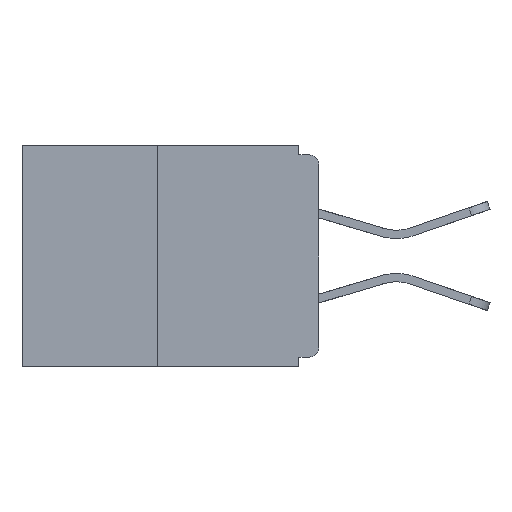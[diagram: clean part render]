
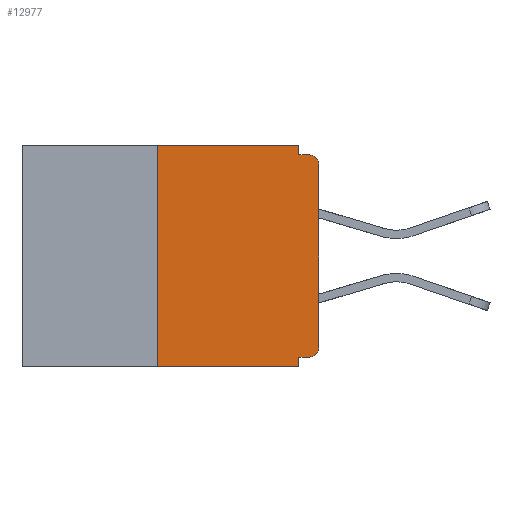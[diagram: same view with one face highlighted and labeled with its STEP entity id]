
A CAD part, left-side view. The second image highlights one B-rep face of the part: STEP entity #12977.
In plain terms, the highlighted planar face has unit normal (-1, 0, 0).
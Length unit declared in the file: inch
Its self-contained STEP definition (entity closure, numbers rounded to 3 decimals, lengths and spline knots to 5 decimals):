
#182 = DIRECTION ( 'NONE',  ( -1., 0., 0. ) ) ;
#202 = CIRCLE ( 'NONE', #8596, 0.015 ) ;
#263 = ORIENTED_EDGE ( 'NONE', *, *, #22919, .T. ) ;
#652 = VERTEX_POINT ( 'NONE', #20610 ) ;
#676 = VERTEX_POINT ( 'NONE', #3017 ) ;
#887 = CARTESIAN_POINT ( 'NONE',  ( 0., 0.031, -0.343 ) ) ;
#1121 = CARTESIAN_POINT ( 'NONE',  ( 0., 0.25, 0. ) ) ;
#1158 = CARTESIAN_POINT ( 'NONE',  ( 0., 0.031, -0.343 ) ) ;
#1607 = VERTEX_POINT ( 'NONE', #1121 ) ;
#2132 = DIRECTION ( 'NONE',  ( -1., 0., 0. ) ) ;
#2192 = VECTOR ( 'NONE', #4013, 39.37008 ) ;
#2248 = ORIENTED_EDGE ( 'NONE', *, *, #24231, .F. ) ;
#2489 = LINE ( 'NONE', #22765, #22977 ) ;
#2720 = VERTEX_POINT ( 'NONE', #15663 ) ;
#2823 = VERTEX_POINT ( 'NONE', #17191 ) ;
#3009 = DIRECTION ( 'NONE',  ( 0., 0., -1. ) ) ;
#3017 = CARTESIAN_POINT ( 'NONE',  ( 0., 0.031, -0.328 ) ) ;
#3618 = LINE ( 'NONE', #21144, #23528 ) ;
#4013 = DIRECTION ( 'NONE',  ( 0., 1., 0. ) ) ;
#4176 = DIRECTION ( 'NONE',  ( 0., -1., 0. ) ) ;
#4643 = VERTEX_POINT ( 'NONE', #14432 ) ;
#5268 = LINE ( 'NONE', #6237, #23670 ) ;
#5896 = ORIENTED_EDGE ( 'NONE', *, *, #14411, .F. ) ;
#6237 = CARTESIAN_POINT ( 'NONE',  ( 0., 0.031, 0. ) ) ;
#6320 = ORIENTED_EDGE ( 'NONE', *, *, #21836, .T. ) ;
#6542 = DIRECTION ( 'NONE',  ( 0., 0., -1. ) ) ;
#6616 = PLANE ( 'NONE',  #24752 ) ;
#7082 = LINE ( 'NONE', #15907, #23379 ) ;
#7353 = CARTESIAN_POINT ( 'NONE',  ( 0., 0.46, 0. ) ) ;
#7375 = VERTEX_POINT ( 'NONE', #23966 ) ;
#7377 = LINE ( 'NONE', #19166, #24196 ) ;
#7943 = DIRECTION ( 'NONE',  ( 0., 0., -1. ) ) ;
#7970 = EDGE_CURVE ( 'NONE', #4643, #1607, #2489, .T. ) ;
#8152 = LINE ( 'NONE', #1158, #17791 ) ;
#8422 = ORIENTED_EDGE ( 'NONE', *, *, #22274, .F. ) ;
#8554 = DIRECTION ( 'NONE',  ( 1., 0., 0. ) ) ;
#8596 = AXIS2_PLACEMENT_3D ( 'NONE', #21632, #2132, #7943 ) ;
#9411 = EDGE_CURVE ( 'NONE', #676, #18682, #8152, .T. ) ;
#10664 = VERTEX_POINT ( 'NONE', #11056 ) ;
#11056 = CARTESIAN_POINT ( 'NONE',  ( 0., 0., -0.03 ) ) ;
#11621 = ORIENTED_EDGE ( 'NONE', *, *, #9411, .F. ) ;
#11983 = FACE_OUTER_BOUND ( 'NONE', #19455, .T. ) ;
#12192 = CARTESIAN_POINT ( 'NONE',  ( 0., 0.015, -0.328 ) ) ;
#12699 = DIRECTION ( 'NONE',  ( 0., -1., 0. ) ) ;
#12977 = ADVANCED_FACE ( 'NONE', ( #11983 ), #6616, .F. ) ;
#13594 = DIRECTION ( 'NONE',  ( 0., -1., 0. ) ) ;
#13879 = DIRECTION ( 'NONE',  ( 0., 0., -1. ) ) ;
#14411 = EDGE_CURVE ( 'NONE', #1607, #2720, #22792, .T. ) ;
#14432 = CARTESIAN_POINT ( 'NONE',  ( 0., 0.25, -0.343 ) ) ;
#15440 = DIRECTION ( 'NONE',  ( 0., 0., 1. ) ) ;
#15663 = CARTESIAN_POINT ( 'NONE',  ( 0., 0.031, 0. ) ) ;
#15907 = CARTESIAN_POINT ( 'NONE',  ( 0., 0., -0.015 ) ) ;
#16020 = AXIS2_PLACEMENT_3D ( 'NONE', #17445, #182, #23494 ) ;
#17191 = CARTESIAN_POINT ( 'NONE',  ( 0., 0.015, -0.015 ) ) ;
#17396 = VECTOR ( 'NONE', #12699, 39.37008 ) ;
#17445 = CARTESIAN_POINT ( 'NONE',  ( 0., 0.015, -0.313 ) ) ;
#17791 = VECTOR ( 'NONE', #3009, 39.37008 ) ;
#18682 = VERTEX_POINT ( 'NONE', #887 ) ;
#19166 = CARTESIAN_POINT ( 'NONE',  ( 0., 0.46, -0.343 ) ) ;
#19455 = EDGE_LOOP ( 'NONE', ( #5896, #22480, #263, #11621, #2248, #20048, #23774, #6320, #20461, #8422 ) ) ;
#20048 = ORIENTED_EDGE ( 'NONE', *, *, #20972, .T. ) ;
#20402 = CIRCLE ( 'NONE', #16020, 0.015 ) ;
#20461 = ORIENTED_EDGE ( 'NONE', *, *, #22398, .F. ) ;
#20610 = CARTESIAN_POINT ( 'NONE',  ( 0., 0.031, -0.015 ) ) ;
#20972 = EDGE_CURVE ( 'NONE', #22016, #7375, #20402, .T. ) ;
#21144 = CARTESIAN_POINT ( 'NONE',  ( 0., 0., 0. ) ) ;
#21451 = CARTESIAN_POINT ( 'NONE',  ( 0., 0., -0.328 ) ) ;
#21632 = CARTESIAN_POINT ( 'NONE',  ( 0., 0.015, -0.03 ) ) ;
#21836 = EDGE_CURVE ( 'NONE', #10664, #2823, #202, .T. ) ;
#22016 = VERTEX_POINT ( 'NONE', #12192 ) ;
#22023 = LINE ( 'NONE', #21451, #2192 ) ;
#22274 = EDGE_CURVE ( 'NONE', #2720, #652, #5268, .T. ) ;
#22398 = EDGE_CURVE ( 'NONE', #652, #2823, #7082, .T. ) ;
#22480 = ORIENTED_EDGE ( 'NONE', *, *, #7970, .F. ) ;
#22765 = CARTESIAN_POINT ( 'NONE',  ( 0., 0.25, 0. ) ) ;
#22792 = LINE ( 'NONE', #7353, #17396 ) ;
#22919 = EDGE_CURVE ( 'NONE', #4643, #18682, #7377, .T. ) ;
#22977 = VECTOR ( 'NONE', #24427, 39.37008 ) ;
#23379 = VECTOR ( 'NONE', #4176, 39.37008 ) ;
#23494 = DIRECTION ( 'NONE',  ( 0., 0., -1. ) ) ;
#23528 = VECTOR ( 'NONE', #15440, 39.37008 ) ;
#23670 = VECTOR ( 'NONE', #13879, 39.37008 ) ;
#23774 = ORIENTED_EDGE ( 'NONE', *, *, #24828, .T. ) ;
#23947 = CARTESIAN_POINT ( 'NONE',  ( 0., 0.46, 0. ) ) ;
#23966 = CARTESIAN_POINT ( 'NONE',  ( 0., 0., -0.313 ) ) ;
#24196 = VECTOR ( 'NONE', #13594, 39.37008 ) ;
#24231 = EDGE_CURVE ( 'NONE', #22016, #676, #22023, .T. ) ;
#24427 = DIRECTION ( 'NONE',  ( 0., 0., 1. ) ) ;
#24752 = AXIS2_PLACEMENT_3D ( 'NONE', #23947, #8554, #6542 ) ;
#24828 = EDGE_CURVE ( 'NONE', #7375, #10664, #3618, .T. ) ;
